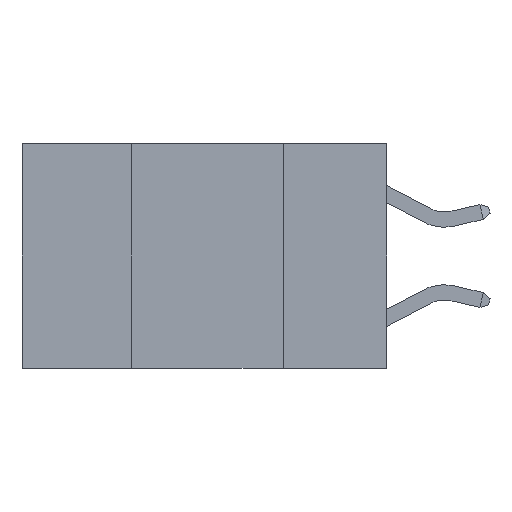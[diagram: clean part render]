
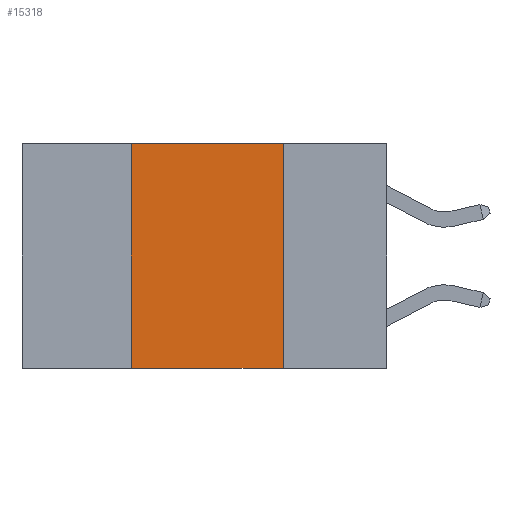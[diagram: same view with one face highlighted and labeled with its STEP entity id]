
A CAD part, left-side view. The second image highlights one B-rep face of the part: STEP entity #15318.
In plain terms, the highlighted planar face has unit normal (-1, 0, 0).
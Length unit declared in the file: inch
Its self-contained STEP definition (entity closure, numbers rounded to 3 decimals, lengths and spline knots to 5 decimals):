
#196 = LINE ( 'NONE', #16889, #10657 ) ;
#346 = VECTOR ( 'NONE', #21690, 39.37008 ) ;
#415 = EDGE_CURVE ( 'NONE', #20829, #16111, #512, .T. ) ;
#512 = LINE ( 'NONE', #20106, #25305 ) ;
#2728 = CARTESIAN_POINT ( 'NONE',  ( 0., 0.17, 0. ) ) ;
#3051 = EDGE_CURVE ( 'NONE', #20591, #13467, #11584, .T. ) ;
#4045 = EDGE_LOOP ( 'NONE', ( #8458, #24748, #12424, #5509 ) ) ;
#4148 = DIRECTION ( 'NONE',  ( 0., 0., 1. ) ) ;
#5182 = CARTESIAN_POINT ( 'NONE',  ( 0., 0.17, -0.37 ) ) ;
#5509 = ORIENTED_EDGE ( 'NONE', *, *, #15338, .T. ) ;
#6044 = PLANE ( 'NONE',  #21012 ) ;
#7920 = CARTESIAN_POINT ( 'NONE',  ( 0., 0.42, -0.37 ) ) ;
#8458 = ORIENTED_EDGE ( 'NONE', *, *, #3051, .F. ) ;
#8649 = VECTOR ( 'NONE', #14340, 39.37008 ) ;
#10578 = CARTESIAN_POINT ( 'NONE',  ( 0., 0.6, 0. ) ) ;
#10657 = VECTOR ( 'NONE', #25507, 39.37008 ) ;
#11584 = LINE ( 'NONE', #13391, #346 ) ;
#12424 = ORIENTED_EDGE ( 'NONE', *, *, #415, .F. ) ;
#13391 = CARTESIAN_POINT ( 'NONE',  ( 0., 0.17, 0. ) ) ;
#13467 = VERTEX_POINT ( 'NONE', #5182 ) ;
#14340 = DIRECTION ( 'NONE',  ( 0., -1., 0. ) ) ;
#15318 = ADVANCED_FACE ( 'NONE', ( #15533 ), #6044, .F. ) ;
#15338 = EDGE_CURVE ( 'NONE', #20829, #13467, #196, .T. ) ;
#15533 = FACE_OUTER_BOUND ( 'NONE', #4045, .T. ) ;
#16111 = VERTEX_POINT ( 'NONE', #17152 ) ;
#16889 = CARTESIAN_POINT ( 'NONE',  ( 0., 0.6, -0.37 ) ) ;
#16981 = EDGE_CURVE ( 'NONE', #16111, #20591, #24059, .T. ) ;
#17152 = CARTESIAN_POINT ( 'NONE',  ( 0., 0.42, 0. ) ) ;
#17746 = DIRECTION ( 'NONE',  ( 1., 0., 0. ) ) ;
#20106 = CARTESIAN_POINT ( 'NONE',  ( 0., 0.42, 0. ) ) ;
#20591 = VERTEX_POINT ( 'NONE', #2728 ) ;
#20829 = VERTEX_POINT ( 'NONE', #7920 ) ;
#21012 = AXIS2_PLACEMENT_3D ( 'NONE', #23434, #17746, #23568 ) ;
#21690 = DIRECTION ( 'NONE',  ( 0., 0., -1. ) ) ;
#23434 = CARTESIAN_POINT ( 'NONE',  ( 0., 0.6, 0. ) ) ;
#23568 = DIRECTION ( 'NONE',  ( 0., 0., -1. ) ) ;
#24059 = LINE ( 'NONE', #10578, #8649 ) ;
#24748 = ORIENTED_EDGE ( 'NONE', *, *, #16981, .F. ) ;
#25305 = VECTOR ( 'NONE', #4148, 39.37008 ) ;
#25507 = DIRECTION ( 'NONE',  ( 0., -1., 0. ) ) ;
